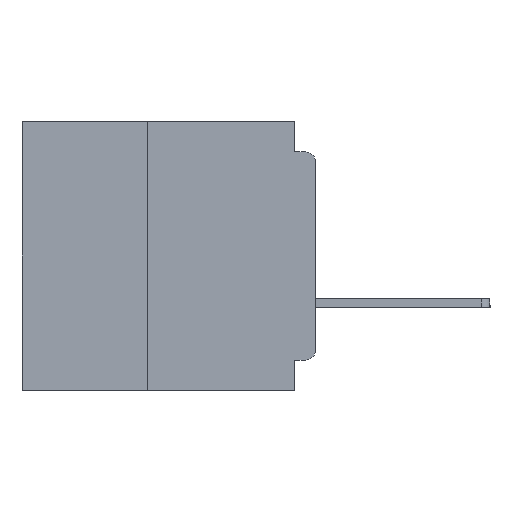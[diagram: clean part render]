
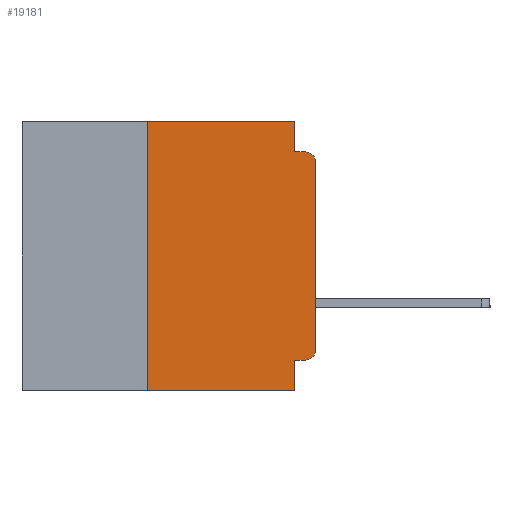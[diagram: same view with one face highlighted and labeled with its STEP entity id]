
A CAD part, left-side view. The second image highlights one B-rep face of the part: STEP entity #19181.
In plain terms, the highlighted planar face has unit normal (-1, 0, 0).
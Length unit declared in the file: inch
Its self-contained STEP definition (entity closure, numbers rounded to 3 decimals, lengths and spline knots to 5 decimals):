
#72 = LINE ( 'NONE', #30613, #9400 ) ;
#126 = ORIENTED_EDGE ( 'NONE', *, *, #27013, .F. ) ;
#845 = CIRCLE ( 'NONE', #40136, 0.015 ) ;
#848 = CARTESIAN_POINT ( 'NONE',  ( 0., 0., -0.34 ) ) ;
#1118 = EDGE_CURVE ( 'NONE', #2477, #13911, #39981, .T. ) ;
#1129 = CARTESIAN_POINT ( 'NONE',  ( 0., 0.015, -0.34 ) ) ;
#1427 = CARTESIAN_POINT ( 'NONE',  ( 0., 0., 0. ) ) ;
#1444 = LINE ( 'NONE', #46099, #10779 ) ;
#1601 = VERTEX_POINT ( 'NONE', #31544 ) ;
#1604 = DIRECTION ( 'NONE',  ( 0., 0., 1. ) ) ;
#2130 = VERTEX_POINT ( 'NONE', #50818 ) ;
#2477 = VERTEX_POINT ( 'NONE', #848 ) ;
#2559 = DIRECTION ( 'NONE',  ( 0., -1., 0. ) ) ;
#4439 = ORIENTED_EDGE ( 'NONE', *, *, #39890, .F. ) ;
#5032 = VECTOR ( 'NONE', #2559, 39.37008 ) ;
#5138 = DIRECTION ( 'NONE',  ( 0., 0., -1. ) ) ;
#5703 = CARTESIAN_POINT ( 'NONE',  ( 0., 0.031, -0.4 ) ) ;
#5722 = CARTESIAN_POINT ( 'NONE',  ( 0., 0.437, 0. ) ) ;
#6114 = ORIENTED_EDGE ( 'NONE', *, *, #35502, .F. ) ;
#6529 = CARTESIAN_POINT ( 'NONE',  ( 0., 0.437, -0.4 ) ) ;
#6758 = CARTESIAN_POINT ( 'NONE',  ( 0., 0.015, -0.06 ) ) ;
#7579 = DIRECTION ( 'NONE',  ( 0., 0., 1. ) ) ;
#7758 = EDGE_CURVE ( 'NONE', #2130, #47980, #1444, .T. ) ;
#8098 = EDGE_LOOP ( 'NONE', ( #14713, #42762, #126, #4439, #6114, #11793, #13800, #10848, #25338, #26109 ) ) ;
#8225 = EDGE_CURVE ( 'NONE', #47980, #17043, #20049, .T. ) ;
#8914 = CARTESIAN_POINT ( 'NONE',  ( 0., 0., -0.06 ) ) ;
#9400 = VECTOR ( 'NONE', #10989, 39.37008 ) ;
#9576 = LINE ( 'NONE', #6529, #29339 ) ;
#10764 = DIRECTION ( 'NONE',  ( 0., 0., -1. ) ) ;
#10779 = VECTOR ( 'NONE', #26521, 39.37008 ) ;
#10848 = ORIENTED_EDGE ( 'NONE', *, *, #8225, .F. ) ;
#10989 = DIRECTION ( 'NONE',  ( 0., 0., -1. ) ) ;
#11428 = CARTESIAN_POINT ( 'NONE',  ( 0., 0.25, -0.4 ) ) ;
#11793 = ORIENTED_EDGE ( 'NONE', *, *, #37261, .F. ) ;
#11971 = VECTOR ( 'NONE', #29372, 39.37008 ) ;
#13498 = CARTESIAN_POINT ( 'NONE',  ( 0., 0.25, 0. ) ) ;
#13560 = EDGE_CURVE ( 'NONE', #13676, #17043, #9576, .T. ) ;
#13676 = VERTEX_POINT ( 'NONE', #15210 ) ;
#13800 = ORIENTED_EDGE ( 'NONE', *, *, #13560, .T. ) ;
#13911 = VERTEX_POINT ( 'NONE', #8914 ) ;
#14713 = ORIENTED_EDGE ( 'NONE', *, *, #1118, .T. ) ;
#15210 = CARTESIAN_POINT ( 'NONE',  ( 0., 0.25, -0.4 ) ) ;
#16177 = VECTOR ( 'NONE', #24046, 39.37008 ) ;
#16760 = EDGE_CURVE ( 'NONE', #13911, #1601, #32701, .T. ) ;
#17043 = VERTEX_POINT ( 'NONE', #43662 ) ;
#17740 = DIRECTION ( 'NONE',  ( 1., 0., 0. ) ) ;
#19181 = ADVANCED_FACE ( 'NONE', ( #50320 ), #21522, .F. ) ;
#19421 = AXIS2_PLACEMENT_3D ( 'NONE', #5722, #17740, #45065 ) ;
#20049 = LINE ( 'NONE', #5703, #11971 ) ;
#20107 = CARTESIAN_POINT ( 'NONE',  ( 0., 0.437, 0. ) ) ;
#21522 = PLANE ( 'NONE',  #19421 ) ;
#22346 = VERTEX_POINT ( 'NONE', #13498 ) ;
#22608 = CARTESIAN_POINT ( 'NONE',  ( 0., 0.031, -0.045 ) ) ;
#24046 = DIRECTION ( 'NONE',  ( 0., -1., 0. ) ) ;
#25214 = VERTEX_POINT ( 'NONE', #22608 ) ;
#25338 = ORIENTED_EDGE ( 'NONE', *, *, #7758, .F. ) ;
#26109 = ORIENTED_EDGE ( 'NONE', *, *, #33481, .T. ) ;
#26521 = DIRECTION ( 'NONE',  ( 0., 1., 0. ) ) ;
#27013 = EDGE_CURVE ( 'NONE', #25214, #1601, #35225, .T. ) ;
#28124 = CARTESIAN_POINT ( 'NONE',  ( 0., 0.031, 0. ) ) ;
#28813 = DIRECTION ( 'NONE',  ( -1., 0., 0. ) ) ;
#29013 = VERTEX_POINT ( 'NONE', #28124 ) ;
#29153 = CARTESIAN_POINT ( 'NONE',  ( 0., 0.031, -0.355 ) ) ;
#29339 = VECTOR ( 'NONE', #34072, 39.37008 ) ;
#29372 = DIRECTION ( 'NONE',  ( 0., 0., -1. ) ) ;
#30102 = AXIS2_PLACEMENT_3D ( 'NONE', #6758, #34302, #10764 ) ;
#30613 = CARTESIAN_POINT ( 'NONE',  ( 0., 0.031, 0. ) ) ;
#31544 = CARTESIAN_POINT ( 'NONE',  ( 0., 0.015, -0.045 ) ) ;
#32701 = CIRCLE ( 'NONE', #30102, 0.015 ) ;
#33481 = EDGE_CURVE ( 'NONE', #2130, #2477, #845, .T. ) ;
#34072 = DIRECTION ( 'NONE',  ( 0., -1., 0. ) ) ;
#34302 = DIRECTION ( 'NONE',  ( -1., 0., 0. ) ) ;
#35225 = LINE ( 'NONE', #41962, #5032 ) ;
#35502 = EDGE_CURVE ( 'NONE', #22346, #29013, #46145, .T. ) ;
#35556 = VECTOR ( 'NONE', #7579, 39.37008 ) ;
#37261 = EDGE_CURVE ( 'NONE', #13676, #22346, #47156, .T. ) ;
#38747 = VECTOR ( 'NONE', #1604, 39.37008 ) ;
#39890 = EDGE_CURVE ( 'NONE', #29013, #25214, #72, .T. ) ;
#39981 = LINE ( 'NONE', #1427, #38747 ) ;
#40136 = AXIS2_PLACEMENT_3D ( 'NONE', #1129, #28813, #5138 ) ;
#41962 = CARTESIAN_POINT ( 'NONE',  ( 0., 0., -0.045 ) ) ;
#42762 = ORIENTED_EDGE ( 'NONE', *, *, #16760, .T. ) ;
#43662 = CARTESIAN_POINT ( 'NONE',  ( 0., 0.031, -0.4 ) ) ;
#45065 = DIRECTION ( 'NONE',  ( 0., 0., -1. ) ) ;
#46099 = CARTESIAN_POINT ( 'NONE',  ( 0., 0., -0.355 ) ) ;
#46145 = LINE ( 'NONE', #20107, #16177 ) ;
#47156 = LINE ( 'NONE', #11428, #35556 ) ;
#47980 = VERTEX_POINT ( 'NONE', #29153 ) ;
#50320 = FACE_OUTER_BOUND ( 'NONE', #8098, .T. ) ;
#50818 = CARTESIAN_POINT ( 'NONE',  ( 0., 0.015, -0.355 ) ) ;
